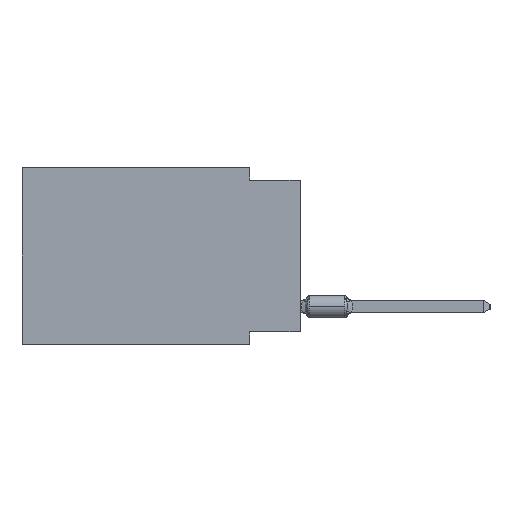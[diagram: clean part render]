
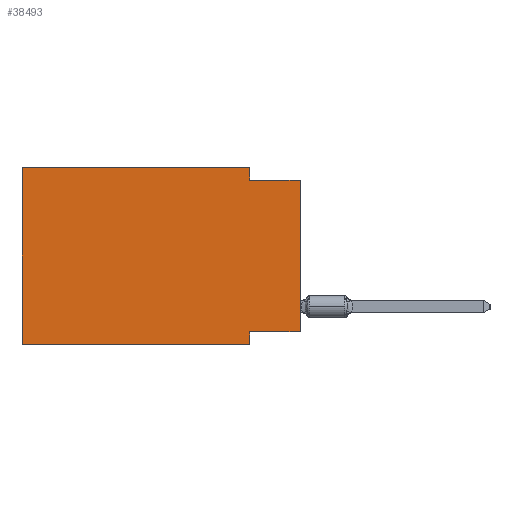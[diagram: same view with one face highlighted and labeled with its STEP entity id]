
A CAD part, left-side view. The second image highlights one B-rep face of the part: STEP entity #38493.
In plain terms, the highlighted planar face has unit normal (-1, 0, 0).
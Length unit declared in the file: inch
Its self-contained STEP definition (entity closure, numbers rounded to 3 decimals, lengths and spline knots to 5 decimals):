
#1006 = ORIENTED_EDGE ( 'NONE', *, *, #39608, .F. ) ;
#1322 = CARTESIAN_POINT ( 'NONE',  ( 0., 0.55, 0. ) ) ;
#2045 = DIRECTION ( 'NONE',  ( 0., 0., -1. ) ) ;
#2059 = CARTESIAN_POINT ( 'NONE',  ( 0., 0.1, 0. ) ) ;
#2616 = DIRECTION ( 'NONE',  ( 0., 0., 1. ) ) ;
#5492 = VERTEX_POINT ( 'NONE', #55771 ) ;
#5565 = AXIS2_PLACEMENT_3D ( 'NONE', #25387, #25689, #7577 ) ;
#5761 = VECTOR ( 'NONE', #21633, 39.37008 ) ;
#5864 = ORIENTED_EDGE ( 'NONE', *, *, #27119, .F. ) ;
#6184 = VECTOR ( 'NONE', #2616, 39.37008 ) ;
#6648 = PLANE ( 'NONE',  #5565 ) ;
#7577 = DIRECTION ( 'NONE',  ( 0., 0., -1. ) ) ;
#8319 = CARTESIAN_POINT ( 'NONE',  ( 0., 0.1, -0.35 ) ) ;
#8369 = VERTEX_POINT ( 'NONE', #31160 ) ;
#8713 = VERTEX_POINT ( 'NONE', #2059 ) ;
#9544 = VECTOR ( 'NONE', #2045, 39.37008 ) ;
#10254 = ORIENTED_EDGE ( 'NONE', *, *, #56697, .F. ) ;
#11943 = CARTESIAN_POINT ( 'NONE',  ( 0., 0., -0.325 ) ) ;
#13078 = ORIENTED_EDGE ( 'NONE', *, *, #39826, .F. ) ;
#13188 = CARTESIAN_POINT ( 'NONE',  ( 0., 0.1, -0.025 ) ) ;
#14438 = DIRECTION ( 'NONE',  ( 0., 0., -1. ) ) ;
#15441 = LINE ( 'NONE', #30118, #39370 ) ;
#16021 = LINE ( 'NONE', #44505, #26561 ) ;
#16638 = LINE ( 'NONE', #41044, #6184 ) ;
#16816 = VECTOR ( 'NONE', #53796, 39.37008 ) ;
#19278 = VERTEX_POINT ( 'NONE', #11943 ) ;
#19999 = VERTEX_POINT ( 'NONE', #21046 ) ;
#20080 = CARTESIAN_POINT ( 'NONE',  ( 0., 0.55, -0.35 ) ) ;
#21046 = CARTESIAN_POINT ( 'NONE',  ( 0., 0.1, -0.325 ) ) ;
#21305 = FACE_OUTER_BOUND ( 'NONE', #56925, .T. ) ;
#21633 = DIRECTION ( 'NONE',  ( 0., -1., 0. ) ) ;
#23560 = VECTOR ( 'NONE', #36809, 39.37008 ) ;
#24664 = ORIENTED_EDGE ( 'NONE', *, *, #35560, .F. ) ;
#25382 = EDGE_CURVE ( 'NONE', #8713, #27247, #49222, .T. ) ;
#25387 = CARTESIAN_POINT ( 'NONE',  ( 0., 0.55, 0. ) ) ;
#25689 = DIRECTION ( 'NONE',  ( 1., 0., 0. ) ) ;
#26561 = VECTOR ( 'NONE', #49488, 39.37008 ) ;
#27119 = EDGE_CURVE ( 'NONE', #5492, #8713, #41348, .T. ) ;
#27247 = VERTEX_POINT ( 'NONE', #13188 ) ;
#29251 = CARTESIAN_POINT ( 'NONE',  ( 0., 0.1, 0. ) ) ;
#29605 = VERTEX_POINT ( 'NONE', #20080 ) ;
#29741 = LINE ( 'NONE', #1322, #16816 ) ;
#30118 = CARTESIAN_POINT ( 'NONE',  ( 0., 0., -0.025 ) ) ;
#31160 = CARTESIAN_POINT ( 'NONE',  ( 0., 0., -0.025 ) ) ;
#33543 = ORIENTED_EDGE ( 'NONE', *, *, #61681, .T. ) ;
#35560 = EDGE_CURVE ( 'NONE', #27247, #8369, #15441, .T. ) ;
#35855 = ORIENTED_EDGE ( 'NONE', *, *, #51884, .T. ) ;
#36630 = CARTESIAN_POINT ( 'NONE',  ( 0., 0.55, 0. ) ) ;
#36809 = DIRECTION ( 'NONE',  ( 0., -1., 0. ) ) ;
#38493 = ADVANCED_FACE ( 'NONE', ( #21305 ), #6648, .F. ) ;
#38505 = LINE ( 'NONE', #56952, #56583 ) ;
#39370 = VECTOR ( 'NONE', #49498, 39.37008 ) ;
#39608 = EDGE_CURVE ( 'NONE', #19278, #19999, #16021, .T. ) ;
#39826 = EDGE_CURVE ( 'NONE', #19999, #42400, #38505, .T. ) ;
#41044 = CARTESIAN_POINT ( 'NONE',  ( 0., 0., 0. ) ) ;
#41218 = LINE ( 'NONE', #41828, #23560 ) ;
#41348 = LINE ( 'NONE', #36630, #5761 ) ;
#41828 = CARTESIAN_POINT ( 'NONE',  ( 0., 0.55, -0.35 ) ) ;
#41878 = ORIENTED_EDGE ( 'NONE', *, *, #25382, .F. ) ;
#42400 = VERTEX_POINT ( 'NONE', #8319 ) ;
#44505 = CARTESIAN_POINT ( 'NONE',  ( 0., 0., -0.325 ) ) ;
#49222 = LINE ( 'NONE', #29251, #9544 ) ;
#49488 = DIRECTION ( 'NONE',  ( 0., 1., 0. ) ) ;
#49498 = DIRECTION ( 'NONE',  ( 0., -1., 0. ) ) ;
#51884 = EDGE_CURVE ( 'NONE', #29605, #42400, #41218, .T. ) ;
#53796 = DIRECTION ( 'NONE',  ( 0., 0., 1. ) ) ;
#55771 = CARTESIAN_POINT ( 'NONE',  ( 0., 0.55, 0. ) ) ;
#56583 = VECTOR ( 'NONE', #14438, 39.37008 ) ;
#56697 = EDGE_CURVE ( 'NONE', #29605, #5492, #29741, .T. ) ;
#56925 = EDGE_LOOP ( 'NONE', ( #33543, #24664, #41878, #5864, #10254, #35855, #13078, #1006 ) ) ;
#56952 = CARTESIAN_POINT ( 'NONE',  ( 0., 0.1, -0.35 ) ) ;
#61681 = EDGE_CURVE ( 'NONE', #19278, #8369, #16638, .T. ) ;
